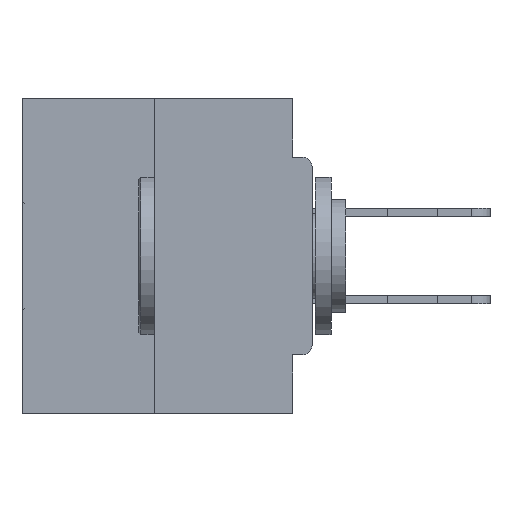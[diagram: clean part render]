
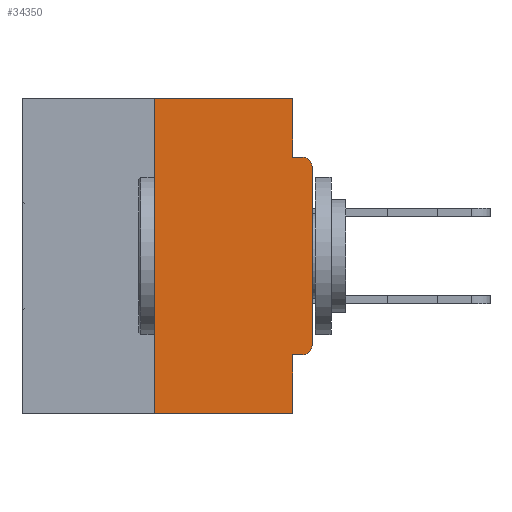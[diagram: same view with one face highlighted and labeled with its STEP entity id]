
A CAD part, left-side view. The second image highlights one B-rep face of the part: STEP entity #34350.
In plain terms, the highlighted planar face has unit normal (-1, 0, 0).
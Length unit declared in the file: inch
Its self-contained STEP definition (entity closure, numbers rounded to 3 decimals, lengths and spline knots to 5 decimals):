
#143 = VERTEX_POINT ( 'NONE', #40486 ) ;
#188 = CARTESIAN_POINT ( 'NONE',  ( 0., 0.031, -0.0935 ) ) ;
#1829 = DIRECTION ( 'NONE',  ( 0., 0., 1. ) ) ;
#1924 = DIRECTION ( 'NONE',  ( 0., 0., -1. ) ) ;
#2156 = VECTOR ( 'NONE', #1829, 39.37008 ) ;
#2213 = ORIENTED_EDGE ( 'NONE', *, *, #37387, .T. ) ;
#2855 = CARTESIAN_POINT ( 'NONE',  ( 0., 0.031, -0.5 ) ) ;
#4068 = EDGE_CURVE ( 'NONE', #35509, #7290, #22443, .T. ) ;
#4150 = CARTESIAN_POINT ( 'NONE',  ( 0., 0.015, -0.1085 ) ) ;
#6070 = DIRECTION ( 'NONE',  ( 0., 0., -1. ) ) ;
#6555 = DIRECTION ( 'NONE',  ( 0., -1., 0. ) ) ;
#6847 = ORIENTED_EDGE ( 'NONE', *, *, #4068, .F. ) ;
#7097 = DIRECTION ( 'NONE',  ( 0., 1., 0. ) ) ;
#7290 = VERTEX_POINT ( 'NONE', #188 ) ;
#7457 = CARTESIAN_POINT ( 'NONE',  ( 0., 0., 0. ) ) ;
#7761 = ORIENTED_EDGE ( 'NONE', *, *, #9391, .F. ) ;
#7847 = ORIENTED_EDGE ( 'NONE', *, *, #22075, .F. ) ;
#8169 = EDGE_CURVE ( 'NONE', #7290, #30760, #10822, .T. ) ;
#9362 = LINE ( 'NONE', #22677, #34589 ) ;
#9391 = EDGE_CURVE ( 'NONE', #41203, #23729, #26211, .T. ) ;
#10802 = DIRECTION ( 'NONE',  ( 0., 0., 1. ) ) ;
#10822 = LINE ( 'NONE', #21984, #32918 ) ;
#11172 = ORIENTED_EDGE ( 'NONE', *, *, #35635, .T. ) ;
#12327 = DIRECTION ( 'NONE',  ( 0., -1., 0. ) ) ;
#13373 = CARTESIAN_POINT ( 'NONE',  ( 0., 0.031, 0. ) ) ;
#14709 = LINE ( 'NONE', #33746, #25017 ) ;
#15613 = VERTEX_POINT ( 'NONE', #18600 ) ;
#16052 = LINE ( 'NONE', #7457, #33620 ) ;
#16392 = EDGE_CURVE ( 'NONE', #15613, #41203, #14709, .T. ) ;
#16960 = VECTOR ( 'NONE', #6070, 39.37008 ) ;
#18235 = DIRECTION ( 'NONE',  ( 0., 0., -1. ) ) ;
#18600 = CARTESIAN_POINT ( 'NONE',  ( 0., 0.015, -0.4065 ) ) ;
#18816 = DIRECTION ( 'NONE',  ( 0., 0., -1. ) ) ;
#20264 = CARTESIAN_POINT ( 'NONE',  ( 0., 0.015, -0.0935 ) ) ;
#20373 = CIRCLE ( 'NONE', #21261, 0.015 ) ;
#20530 = CARTESIAN_POINT ( 'NONE',  ( 0., 0.46, 0. ) ) ;
#20588 = DIRECTION ( 'NONE',  ( 0., 0., -1. ) ) ;
#20920 = VERTEX_POINT ( 'NONE', #23491 ) ;
#21261 = AXIS2_PLACEMENT_3D ( 'NONE', #4150, #40172, #20588 ) ;
#21585 = EDGE_CURVE ( 'NONE', #15613, #36630, #30616, .T. ) ;
#21943 = VECTOR ( 'NONE', #18235, 39.37008 ) ;
#21984 = CARTESIAN_POINT ( 'NONE',  ( 0., 0., -0.0935 ) ) ;
#22075 = EDGE_CURVE ( 'NONE', #32900, #20920, #40360, .T. ) ;
#22279 = LINE ( 'NONE', #20530, #25381 ) ;
#22443 = LINE ( 'NONE', #31616, #21943 ) ;
#22460 = EDGE_CURVE ( 'NONE', #36630, #143, #16052, .T. ) ;
#22677 = CARTESIAN_POINT ( 'NONE',  ( 0., 0.46, -0.5 ) ) ;
#23491 = CARTESIAN_POINT ( 'NONE',  ( 0., 0.25, 0. ) ) ;
#23729 = VERTEX_POINT ( 'NONE', #25886 ) ;
#23734 = AXIS2_PLACEMENT_3D ( 'NONE', #25287, #28481, #18816 ) ;
#25017 = VECTOR ( 'NONE', #7097, 39.37008 ) ;
#25287 = CARTESIAN_POINT ( 'NONE',  ( 0., 0.46, 0. ) ) ;
#25381 = VECTOR ( 'NONE', #40254, 39.37008 ) ;
#25886 = CARTESIAN_POINT ( 'NONE',  ( 0., 0.031, -0.5 ) ) ;
#26211 = LINE ( 'NONE', #2855, #16960 ) ;
#27086 = CARTESIAN_POINT ( 'NONE',  ( 0., 0., -0.3915 ) ) ;
#28481 = DIRECTION ( 'NONE',  ( 1., 0., 0. ) ) ;
#30616 = CIRCLE ( 'NONE', #31125, 0.015 ) ;
#30760 = VERTEX_POINT ( 'NONE', #20264 ) ;
#30868 = ORIENTED_EDGE ( 'NONE', *, *, #22460, .T. ) ;
#31125 = AXIS2_PLACEMENT_3D ( 'NONE', #38129, #34923, #1924 ) ;
#31616 = CARTESIAN_POINT ( 'NONE',  ( 0., 0.031, 0. ) ) ;
#32900 = VERTEX_POINT ( 'NONE', #38879 ) ;
#32918 = VECTOR ( 'NONE', #12327, 39.37008 ) ;
#33620 = VECTOR ( 'NONE', #10802, 39.37008 ) ;
#33746 = CARTESIAN_POINT ( 'NONE',  ( 0., 0., -0.4065 ) ) ;
#34350 = ADVANCED_FACE ( 'NONE', ( #34861 ), #34922, .F. ) ;
#34589 = VECTOR ( 'NONE', #6555, 39.37008 ) ;
#34861 = FACE_OUTER_BOUND ( 'NONE', #36744, .T. ) ;
#34922 = PLANE ( 'NONE',  #23734 ) ;
#34923 = DIRECTION ( 'NONE',  ( -1., 0., 0. ) ) ;
#35509 = VERTEX_POINT ( 'NONE', #13373 ) ;
#35635 = EDGE_CURVE ( 'NONE', #143, #30760, #20373, .T. ) ;
#35885 = ORIENTED_EDGE ( 'NONE', *, *, #40568, .F. ) ;
#36630 = VERTEX_POINT ( 'NONE', #27086 ) ;
#36744 = EDGE_LOOP ( 'NONE', ( #35885, #7847, #2213, #7761, #38794, #37202, #30868, #11172, #42520, #6847 ) ) ;
#37202 = ORIENTED_EDGE ( 'NONE', *, *, #21585, .T. ) ;
#37387 = EDGE_CURVE ( 'NONE', #32900, #23729, #9362, .T. ) ;
#38129 = CARTESIAN_POINT ( 'NONE',  ( 0., 0.015, -0.3915 ) ) ;
#38305 = CARTESIAN_POINT ( 'NONE',  ( 0., 0.25, 0. ) ) ;
#38794 = ORIENTED_EDGE ( 'NONE', *, *, #16392, .F. ) ;
#38879 = CARTESIAN_POINT ( 'NONE',  ( 0., 0.25, -0.5 ) ) ;
#39820 = CARTESIAN_POINT ( 'NONE',  ( 0., 0.031, -0.4065 ) ) ;
#40172 = DIRECTION ( 'NONE',  ( -1., 0., 0. ) ) ;
#40254 = DIRECTION ( 'NONE',  ( 0., -1., 0. ) ) ;
#40360 = LINE ( 'NONE', #38305, #2156 ) ;
#40486 = CARTESIAN_POINT ( 'NONE',  ( 0., 0., -0.1085 ) ) ;
#40568 = EDGE_CURVE ( 'NONE', #20920, #35509, #22279, .T. ) ;
#41203 = VERTEX_POINT ( 'NONE', #39820 ) ;
#42520 = ORIENTED_EDGE ( 'NONE', *, *, #8169, .F. ) ;
